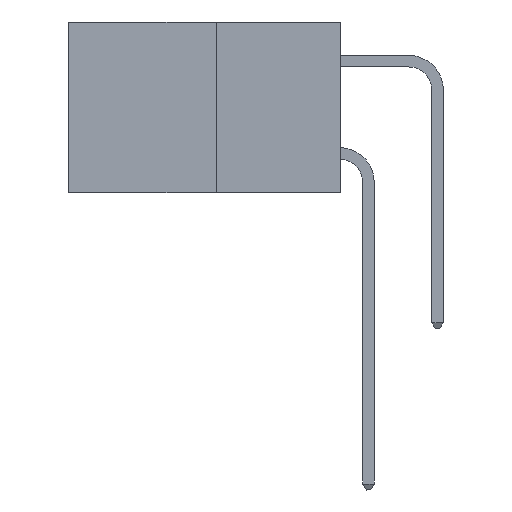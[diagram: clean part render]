
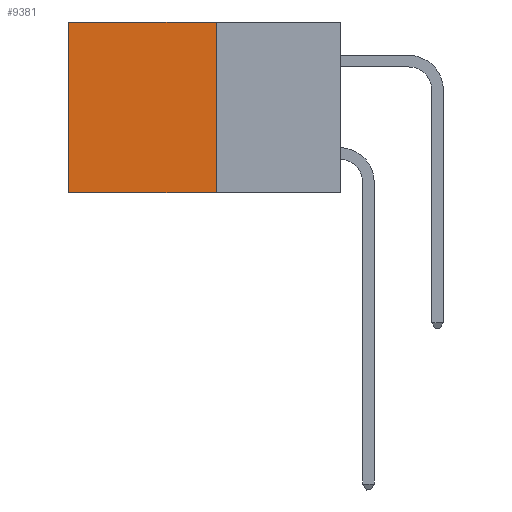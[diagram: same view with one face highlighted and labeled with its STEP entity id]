
A CAD part, left-side view. The second image highlights one B-rep face of the part: STEP entity #9381.
In plain terms, the highlighted planar face has unit normal (-1, 0, 0).
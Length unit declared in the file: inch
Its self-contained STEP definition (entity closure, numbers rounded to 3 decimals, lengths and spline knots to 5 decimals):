
#76 = DIRECTION ( 'NONE',  ( 0., 1., 0. ) ) ;
#1420 = CARTESIAN_POINT ( 'NONE',  ( 0.277, 0.59, 0. ) ) ;
#4354 = VECTOR ( 'NONE', #28525, 39.37008 ) ;
#4902 = PLANE ( 'NONE',  #12460 ) ;
#4995 = EDGE_CURVE ( 'NONE', #26487, #13303, #20062, .T. ) ;
#5094 = CARTESIAN_POINT ( 'NONE',  ( 0.277, 0.27, 0. ) ) ;
#6812 = CARTESIAN_POINT ( 'NONE',  ( 0.277, 0.27, 0. ) ) ;
#7387 = EDGE_CURVE ( 'NONE', #13303, #13977, #13718, .T. ) ;
#7547 = DIRECTION ( 'NONE',  ( 0., 0., -1. ) ) ;
#9381 = ADVANCED_FACE ( 'NONE', ( #19705 ), #4902, .F. ) ;
#11437 = VECTOR ( 'NONE', #23445, 39.37008 ) ;
#12177 = DIRECTION ( 'NONE',  ( 0., 1., 0. ) ) ;
#12460 = AXIS2_PLACEMENT_3D ( 'NONE', #33595, #23311, #7547 ) ;
#12898 = ORIENTED_EDGE ( 'NONE', *, *, #4995, .F. ) ;
#12936 = CARTESIAN_POINT ( 'NONE',  ( 0.277, 0.59, -0.37 ) ) ;
#13303 = VERTEX_POINT ( 'NONE', #31031 ) ;
#13718 = LINE ( 'NONE', #18531, #26757 ) ;
#13846 = EDGE_LOOP ( 'NONE', ( #14713, #15520, #12898, #21912 ) ) ;
#13977 = VERTEX_POINT ( 'NONE', #15289 ) ;
#14713 = ORIENTED_EDGE ( 'NONE', *, *, #32448, .T. ) ;
#15289 = CARTESIAN_POINT ( 'NONE',  ( 0.277, 0.59, -0.37 ) ) ;
#15520 = ORIENTED_EDGE ( 'NONE', *, *, #7387, .F. ) ;
#15917 = LINE ( 'NONE', #6812, #28945 ) ;
#16810 = VERTEX_POINT ( 'NONE', #1420 ) ;
#18531 = CARTESIAN_POINT ( 'NONE',  ( 0.277, 0.27, -0.37 ) ) ;
#19705 = FACE_OUTER_BOUND ( 'NONE', #13846, .T. ) ;
#20062 = LINE ( 'NONE', #27178, #11437 ) ;
#21912 = ORIENTED_EDGE ( 'NONE', *, *, #32952, .T. ) ;
#23311 = DIRECTION ( 'NONE',  ( 1., 0., 0. ) ) ;
#23445 = DIRECTION ( 'NONE',  ( 0., 0., -1. ) ) ;
#25335 = LINE ( 'NONE', #12936, #4354 ) ;
#26487 = VERTEX_POINT ( 'NONE', #5094 ) ;
#26757 = VECTOR ( 'NONE', #76, 39.37008 ) ;
#27178 = CARTESIAN_POINT ( 'NONE',  ( 0.277, 0.27, -0.37 ) ) ;
#28525 = DIRECTION ( 'NONE',  ( 0., 0., -1. ) ) ;
#28945 = VECTOR ( 'NONE', #12177, 39.37008 ) ;
#31031 = CARTESIAN_POINT ( 'NONE',  ( 0.277, 0.27, -0.37 ) ) ;
#32448 = EDGE_CURVE ( 'NONE', #16810, #13977, #25335, .T. ) ;
#32952 = EDGE_CURVE ( 'NONE', #26487, #16810, #15917, .T. ) ;
#33595 = CARTESIAN_POINT ( 'NONE',  ( 0.277, 0.27, -0.37 ) ) ;
